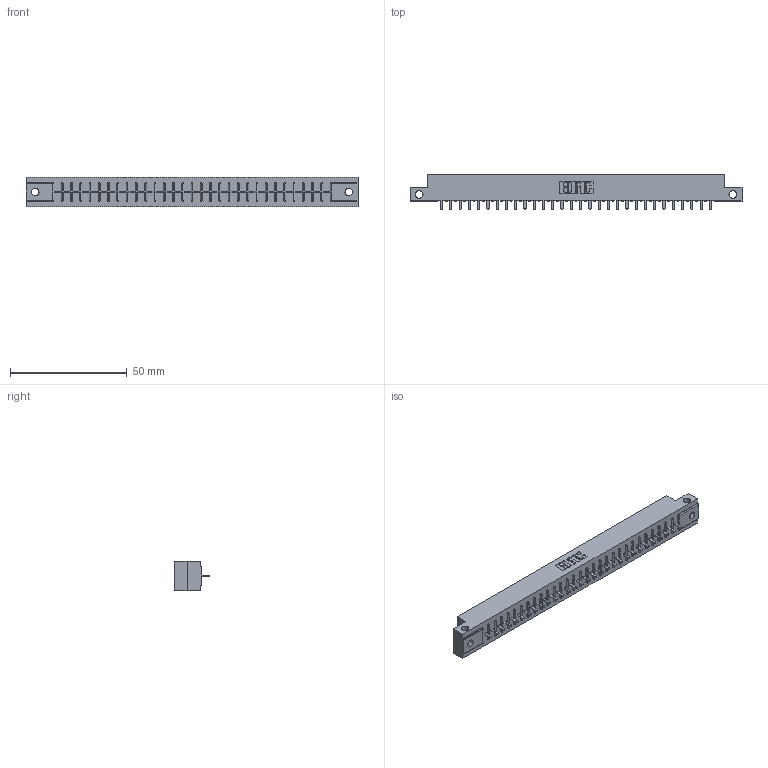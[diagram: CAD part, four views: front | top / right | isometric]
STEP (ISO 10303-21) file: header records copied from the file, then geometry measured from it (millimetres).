
FILE_DESCRIPTION (( 'STEP AP203' ), '1' );
FILE_NAME ('316-030-521-112.STEP', '2020-09-20T21:13:16', ( '' ), ( '' ), 'SwSTEP 2.0', 'SolidWorks 2020', '' );
FILE_SCHEMA (( 'CONFIG_CONTROL_DESIGN' ));
Length unit declared in the file: inch
Products named in the file (3): 306-290-001_121; 316-030-521-112; 306 Part_.128 Dia
Assembly tree (31 placements, depth 2):
  316-030-521-112
    306 Part_.128 Dia
    306-290-001_121  x30
Bounding box: 141.88 x 14.88 x 12.7 mm (x, y, z)
Volume: 15346.1 mm3; surface area: 15426.9 mm2
Topology: 31 solids, 31 shells, 2228 faces, 6262 edges, 4008 vertices
Faces by surface type: plane 1478, cylinder 630, sphere 120
Entity records: 29893 total; most frequent: CARTESIAN_POINT 5065, ORIENTED_EDGE 4976, DIRECTION 4934, EDGE_CURVE 2488, LINE 1924, VECTOR 1924, VERTEX_POINT 1572, AXIS2_PLACEMENT_3D 1505
